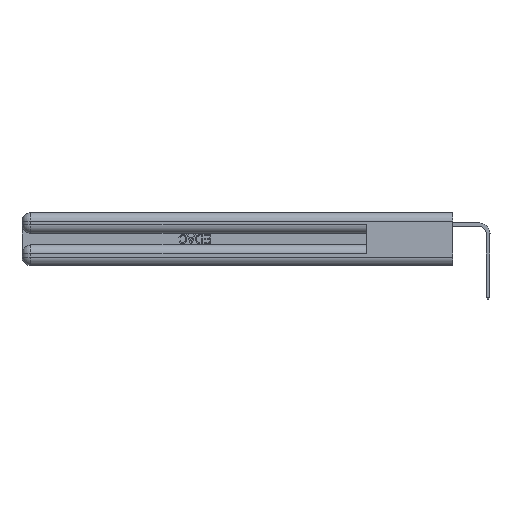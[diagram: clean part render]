
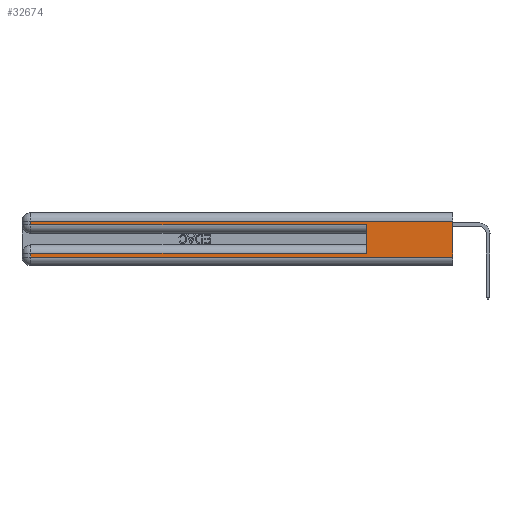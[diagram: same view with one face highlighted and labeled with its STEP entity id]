
A CAD part, left-side view. The second image highlights one B-rep face of the part: STEP entity #32674.
In plain terms, the highlighted planar face has unit normal (-1, 0, 0).
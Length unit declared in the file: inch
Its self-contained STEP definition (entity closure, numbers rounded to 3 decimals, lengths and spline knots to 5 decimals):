
#43 = CARTESIAN_POINT ( 'NONE',  ( 0., 0.6, 0.085 ) ) ;
#1185 = CARTESIAN_POINT ( 'NONE',  ( 0., 0.6, 0.145 ) ) ;
#1459 = VECTOR ( 'NONE', #36920, 39.37008 ) ;
#2886 = ORIENTED_EDGE ( 'NONE', *, *, #37516, .F. ) ;
#3081 = EDGE_CURVE ( 'NONE', #10464, #3317, #44218, .T. ) ;
#3317 = VERTEX_POINT ( 'NONE', #48099 ) ;
#4435 = CARTESIAN_POINT ( 'NONE',  ( 0., 0., 0.06 ) ) ;
#5200 = ORIENTED_EDGE ( 'NONE', *, *, #16762, .T. ) ;
#6124 = VERTEX_POINT ( 'NONE', #18989 ) ;
#7824 = EDGE_CURVE ( 'NONE', #7863, #10464, #30431, .T. ) ;
#7863 = VERTEX_POINT ( 'NONE', #46704 ) ;
#8867 = VERTEX_POINT ( 'NONE', #17278 ) ;
#9066 = ORIENTED_EDGE ( 'NONE', *, *, #23043, .T. ) ;
#9207 = FACE_OUTER_BOUND ( 'NONE', #50707, .T. ) ;
#10464 = VERTEX_POINT ( 'NONE', #11389 ) ;
#11293 = VECTOR ( 'NONE', #50619, 39.37008 ) ;
#11389 = CARTESIAN_POINT ( 'NONE',  ( 0., 2.94, 0.285 ) ) ;
#12545 = PLANE ( 'NONE',  #28050 ) ;
#12618 = CARTESIAN_POINT ( 'NONE',  ( 0., 2.94, 0.06 ) ) ;
#16527 = DIRECTION ( 'NONE',  ( 0., 0., -1. ) ) ;
#16762 = EDGE_CURVE ( 'NONE', #20600, #22596, #33843, .T. ) ;
#17278 = CARTESIAN_POINT ( 'NONE',  ( 0., 0., 0.31 ) ) ;
#18647 = CARTESIAN_POINT ( 'NONE',  ( 0., 2.94, 0.37 ) ) ;
#18989 = CARTESIAN_POINT ( 'NONE',  ( 0., 2.94, 0.085 ) ) ;
#19812 = VECTOR ( 'NONE', #30693, 39.37008 ) ;
#20600 = VERTEX_POINT ( 'NONE', #12618 ) ;
#21755 = VECTOR ( 'NONE', #22852, 39.37008 ) ;
#21994 = VECTOR ( 'NONE', #30439, 39.37008 ) ;
#22596 = VERTEX_POINT ( 'NONE', #4435 ) ;
#22852 = DIRECTION ( 'NONE',  ( 0., -1., 0. ) ) ;
#23043 = EDGE_CURVE ( 'NONE', #8867, #7863, #43105, .T. ) ;
#23245 = LINE ( 'NONE', #26440, #21994 ) ;
#26094 = LINE ( 'NONE', #36650, #44772 ) ;
#26440 = CARTESIAN_POINT ( 'NONE',  ( 0., 2.94, 0.37 ) ) ;
#26790 = LINE ( 'NONE', #33566, #47963 ) ;
#26801 = ORIENTED_EDGE ( 'NONE', *, *, #44328, .T. ) ;
#27079 = ORIENTED_EDGE ( 'NONE', *, *, #3081, .T. ) ;
#28050 = AXIS2_PLACEMENT_3D ( 'NONE', #28454, #40411, #16527 ) ;
#28454 = CARTESIAN_POINT ( 'NONE',  ( 0., 0., 0.37 ) ) ;
#28679 = DIRECTION ( 'NONE',  ( 0., 1., 0. ) ) ;
#29478 = EDGE_CURVE ( 'NONE', #6124, #20600, #23245, .T. ) ;
#29699 = VERTEX_POINT ( 'NONE', #43 ) ;
#30431 = LINE ( 'NONE', #18647, #19812 ) ;
#30439 = DIRECTION ( 'NONE',  ( 0., 0., -1. ) ) ;
#30693 = DIRECTION ( 'NONE',  ( 0., 0., -1. ) ) ;
#32673 = ORIENTED_EDGE ( 'NONE', *, *, #7824, .T. ) ;
#32674 = ADVANCED_FACE ( 'NONE', ( #9207 ), #12545, .F. ) ;
#33566 = CARTESIAN_POINT ( 'NONE',  ( 0., 0., 0.37 ) ) ;
#33843 = LINE ( 'NONE', #41766, #43200 ) ;
#34732 = CARTESIAN_POINT ( 'NONE',  ( 0., 0., 0.31 ) ) ;
#34996 = EDGE_CURVE ( 'NONE', #29699, #3317, #42620, .T. ) ;
#35498 = ORIENTED_EDGE ( 'NONE', *, *, #34996, .F. ) ;
#36650 = CARTESIAN_POINT ( 'NONE',  ( 0., 0., 0.085 ) ) ;
#36920 = DIRECTION ( 'NONE',  ( 0., 0., 1. ) ) ;
#37516 = EDGE_CURVE ( 'NONE', #8867, #22596, #26790, .T. ) ;
#39464 = ORIENTED_EDGE ( 'NONE', *, *, #29478, .T. ) ;
#40411 = DIRECTION ( 'NONE',  ( 1., 0., 0. ) ) ;
#41766 = CARTESIAN_POINT ( 'NONE',  ( 0., 0., 0.06 ) ) ;
#42620 = LINE ( 'NONE', #1185, #1459 ) ;
#43105 = LINE ( 'NONE', #34732, #11293 ) ;
#43200 = VECTOR ( 'NONE', #45820, 39.37008 ) ;
#44218 = LINE ( 'NONE', #50753, #21755 ) ;
#44328 = EDGE_CURVE ( 'NONE', #29699, #6124, #26094, .T. ) ;
#44772 = VECTOR ( 'NONE', #28679, 39.37008 ) ;
#45820 = DIRECTION ( 'NONE',  ( 0., -1., 0. ) ) ;
#46704 = CARTESIAN_POINT ( 'NONE',  ( 0., 2.94, 0.31 ) ) ;
#47963 = VECTOR ( 'NONE', #49627, 39.37008 ) ;
#48099 = CARTESIAN_POINT ( 'NONE',  ( 0., 0.6, 0.285 ) ) ;
#49627 = DIRECTION ( 'NONE',  ( 0., 0., -1. ) ) ;
#50619 = DIRECTION ( 'NONE',  ( 0., 1., 0. ) ) ;
#50707 = EDGE_LOOP ( 'NONE', ( #2886, #9066, #32673, #27079, #35498, #26801, #39464, #5200 ) ) ;
#50753 = CARTESIAN_POINT ( 'NONE',  ( 0., 0., 0.285 ) ) ;
